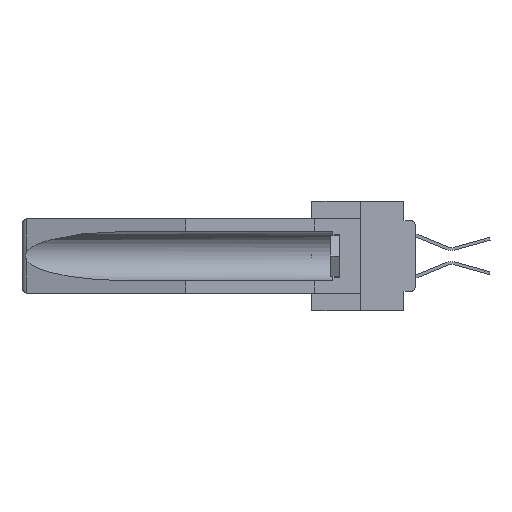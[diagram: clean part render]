
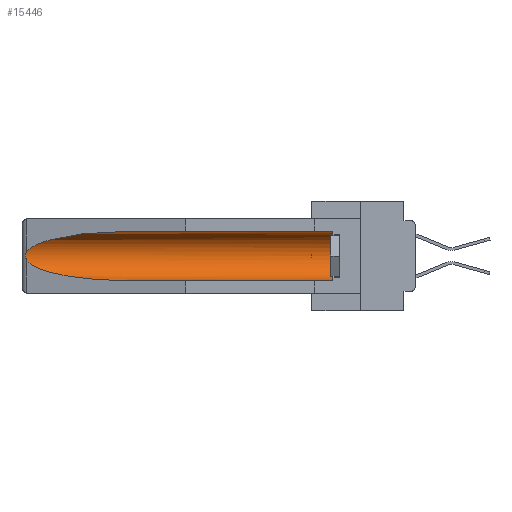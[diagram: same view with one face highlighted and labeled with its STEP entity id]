
A CAD part, left-side view. The second image highlights one B-rep face of the part: STEP entity #15446.
In plain terms, the highlighted cylindrical face has radius 2.857 mm (diameter 5.715 mm), a partial arc.
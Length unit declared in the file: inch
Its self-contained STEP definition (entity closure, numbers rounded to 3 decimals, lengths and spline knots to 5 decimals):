
#116 = CARTESIAN_POINT ( 'NONE',  ( 0.21114, 1.30732, -0.059 ) ) ;
#259 =( BOUNDED_CURVE ( )  B_SPLINE_CURVE ( 3, ( #9403, #116, #12678, #21551 ),
 .UNSPECIFIED., .F., .T. ) 
 B_SPLINE_CURVE_WITH_KNOTS ( ( 4, 4 ),
 ( 4.71239, 6.08839 ),
 .UNSPECIFIED. ) 
 CURVE ( )  GEOMETRIC_REPRESENTATION_ITEM ( )  RATIONAL_B_SPLINE_CURVE ( ( 1., 0.848, 0.848, 1. ) ) 
 REPRESENTATION_ITEM ( '' )  );
#363 = AXIS2_PLACEMENT_3D ( 'NONE', #9991, #13886, #4421 ) ;
#863 = B_SPLINE_CURVE_WITH_KNOTS ( 'NONE', 3,
 ( #1231, #4136, #1433, #16696, #32751, #29266, #14014, #1042, #38731, #19982 ),
 .UNSPECIFIED., .F., .F.,
 ( 4, 2, 2, 2, 4 ),
 ( 0., 0.00029, 0.00058, 0.00087, 0.00117 ),
 .UNSPECIFIED. ) ;
#1042 = CARTESIAN_POINT ( 'NONE',  ( 0.26655, 1.53094, -0.18657 ) ) ;
#1231 = CARTESIAN_POINT ( 'NONE',  ( 0.26537, 1.52718, -0.14972 ) ) ;
#1433 = CARTESIAN_POINT ( 'NONE',  ( 0.26654, 1.53092, -0.15636 ) ) ;
#2488 = CARTESIAN_POINT ( 'NONE',  ( 0.155, 1.07973, -0.284 ) ) ;
#3060 = VECTOR ( 'NONE', #38469, 39.37008 ) ;
#4136 = CARTESIAN_POINT ( 'NONE',  ( 0.26597, 1.52961, -0.15275 ) ) ;
#4421 = DIRECTION ( 'NONE',  ( 0., 0., 1. ) ) ;
#5620 = VERTEX_POINT ( 'NONE', #40256 ) ;
#6525 = ORIENTED_EDGE ( 'NONE', *, *, #27439, .T. ) ;
#6771 = EDGE_CURVE ( 'NONE', #30986, #33028, #33933, .T. ) ;
#7204 = LINE ( 'NONE', #12783, #24931 ) ;
#7782 = CARTESIAN_POINT ( 'NONE',  ( 0.155, 1.07973, -0.284 ) ) ;
#8334 = ORIENTED_EDGE ( 'NONE', *, *, #10828, .T. ) ;
#9010 = CARTESIAN_POINT ( 'NONE',  ( 0.26537, 1.52718, -0.14972 ) ) ;
#9403 = CARTESIAN_POINT ( 'NONE',  ( 0.155, 1.07973, -0.059 ) ) ;
#9991 = CARTESIAN_POINT ( 'NONE',  ( 0.155, 0.126, -0.1715 ) ) ;
#10828 = EDGE_CURVE ( 'NONE', #28449, #23027, #259, .T. ) ;
#10880 = CARTESIAN_POINT ( 'NONE',  ( 0.26537, 1.52718, -0.19328 ) ) ;
#12678 = CARTESIAN_POINT ( 'NONE',  ( 0.25451, 1.48313, -0.09465 ) ) ;
#12783 = CARTESIAN_POINT ( 'NONE',  ( 0.155, -0.30754, -0.284 ) ) ;
#13886 = DIRECTION ( 'NONE',  ( 0., -1., 0. ) ) ;
#14014 = CARTESIAN_POINT ( 'NONE',  ( 0.2673, 1.53269, -0.17917 ) ) ;
#14848 = ORIENTED_EDGE ( 'NONE', *, *, #6771, .T. ) ;
#15446 = ADVANCED_FACE ( 'NONE', ( #31646 ), #21992, .F. ) ;
#16041 = EDGE_CURVE ( 'NONE', #23027, #30986, #863, .T. ) ;
#16286 = ORIENTED_EDGE ( 'NONE', *, *, #16041, .T. ) ;
#16696 = CARTESIAN_POINT ( 'NONE',  ( 0.2673, 1.5327, -0.16383 ) ) ;
#18897 = DIRECTION ( 'NONE',  ( 0., 0., 1. ) ) ;
#19520 = CARTESIAN_POINT ( 'NONE',  ( 0.155, -0.30754, -0.059 ) ) ;
#19982 = CARTESIAN_POINT ( 'NONE',  ( 0.26537, 1.52718, -0.19328 ) ) ;
#21551 = CARTESIAN_POINT ( 'NONE',  ( 0.26537, 1.52718, -0.14972 ) ) ;
#21992 = CYLINDRICAL_SURFACE ( 'NONE', #40379, 0.1125 ) ;
#22381 = DIRECTION ( 'NONE',  ( 0., 1., 0. ) ) ;
#23027 = VERTEX_POINT ( 'NONE', #9010 ) ;
#23437 = CARTESIAN_POINT ( 'NONE',  ( 0.21114, 1.30732, -0.284 ) ) ;
#24396 = CARTESIAN_POINT ( 'NONE',  ( 0.26537, 1.52718, -0.19328 ) ) ;
#24931 = VECTOR ( 'NONE', #37915, 39.37008 ) ;
#25085 = ORIENTED_EDGE ( 'NONE', *, *, #30390, .T. ) ;
#25370 = CIRCLE ( 'NONE', #363, 0.1125 ) ;
#25499 = CARTESIAN_POINT ( 'NONE',  ( 0.155, -0.30754, -0.1715 ) ) ;
#27439 = EDGE_CURVE ( 'NONE', #38518, #5620, #25370, .T. ) ;
#28449 = VERTEX_POINT ( 'NONE', #37978 ) ;
#29266 = CARTESIAN_POINT ( 'NONE',  ( 0.2675, 1.53308, -0.17534 ) ) ;
#30390 = EDGE_CURVE ( 'NONE', #5620, #28449, #36181, .T. ) ;
#30986 = VERTEX_POINT ( 'NONE', #24396 ) ;
#31646 = FACE_OUTER_BOUND ( 'NONE', #35749, .T. ) ;
#32751 = CARTESIAN_POINT ( 'NONE',  ( 0.2675, 1.53308, -0.16763 ) ) ;
#33028 = VERTEX_POINT ( 'NONE', #2488 ) ;
#33874 = CARTESIAN_POINT ( 'NONE',  ( 0.155, 0.126, -0.284 ) ) ;
#33933 =( BOUNDED_CURVE ( )  B_SPLINE_CURVE ( 3, ( #10880, #38688, #23437, #7782 ),
 .UNSPECIFIED., .F., .T. ) 
 B_SPLINE_CURVE_WITH_KNOTS ( ( 4, 4 ),
 ( 0.1948, 1.5708 ),
 .UNSPECIFIED. ) 
 CURVE ( )  GEOMETRIC_REPRESENTATION_ITEM ( )  RATIONAL_B_SPLINE_CURVE ( ( 1., 0.848, 0.848, 1. ) ) 
 REPRESENTATION_ITEM ( '' )  );
#34468 = EDGE_CURVE ( 'NONE', #38518, #33028, #7204, .T. ) ;
#35496 = ORIENTED_EDGE ( 'NONE', *, *, #34468, .F. ) ;
#35749 = EDGE_LOOP ( 'NONE', ( #8334, #16286, #14848, #35496, #6525, #25085 ) ) ;
#36181 = LINE ( 'NONE', #19520, #3060 ) ;
#37915 = DIRECTION ( 'NONE',  ( 0., 1., 0. ) ) ;
#37978 = CARTESIAN_POINT ( 'NONE',  ( 0.155, 1.07973, -0.059 ) ) ;
#38469 = DIRECTION ( 'NONE',  ( 0., 1., 0. ) ) ;
#38518 = VERTEX_POINT ( 'NONE', #33874 ) ;
#38688 = CARTESIAN_POINT ( 'NONE',  ( 0.25451, 1.48313, -0.24835 ) ) ;
#38731 = CARTESIAN_POINT ( 'NONE',  ( 0.26597, 1.5296, -0.19026 ) ) ;
#40256 = CARTESIAN_POINT ( 'NONE',  ( 0.155, 0.126, -0.059 ) ) ;
#40379 = AXIS2_PLACEMENT_3D ( 'NONE', #25499, #22381, #18897 ) ;
